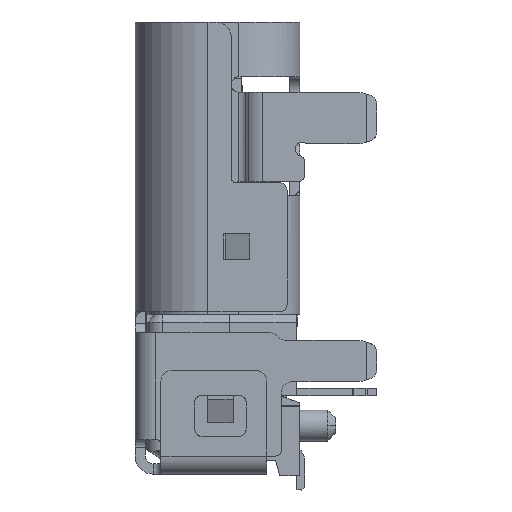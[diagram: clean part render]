
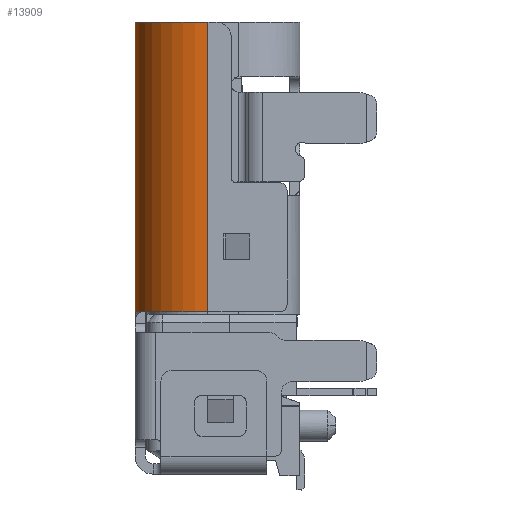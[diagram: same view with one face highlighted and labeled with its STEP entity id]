
A CAD part, left-side view. The second image highlights one B-rep face of the part: STEP entity #13909.
In plain terms, the highlighted cylindrical face has radius 1.41 mm (diameter 2.82 mm), a partial arc.
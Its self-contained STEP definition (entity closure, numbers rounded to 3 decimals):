
#356 = CYLINDRICAL_SURFACE ( 'NONE', #32464, 1.41 ) ;
#725 = CIRCLE ( 'NONE', #54226, 1.41 ) ;
#740 = VECTOR ( 'NONE', #38979, 1000. ) ;
#6155 = ORIENTED_EDGE ( 'NONE', *, *, #52917, .T. ) ;
#6172 = EDGE_CURVE ( 'NONE', #33294, #39685, #14687, .T. ) ;
#8142 = DIRECTION ( 'NONE',  ( 0., 0., 1. ) ) ;
#9703 = ORIENTED_EDGE ( 'NONE', *, *, #45828, .F. ) ;
#11877 = CARTESIAN_POINT ( 'NONE',  ( -360.4, -0.3, -255.061 ) ) ;
#13909 = ADVANCED_FACE ( 'NONE', ( #19484 ), #356, .T. ) ;
#14687 = LINE ( 'NONE', #74076, #740 ) ;
#17367 = LINE ( 'NONE', #78723, #37269 ) ;
#19484 = FACE_OUTER_BOUND ( 'NONE', #42859, .T. ) ;
#20336 = CARTESIAN_POINT ( 'NONE',  ( -361.81, -0.3, -249.451 ) ) ;
#21055 = EDGE_CURVE ( 'NONE', #33294, #36418, #49815, .T. ) ;
#22027 = VERTEX_POINT ( 'NONE', #27323 ) ;
#25680 = DIRECTION ( 'NONE',  ( 1., 0., 0. ) ) ;
#27323 = CARTESIAN_POINT ( 'NONE',  ( -360.4, -0.3, -249.451 ) ) ;
#29666 = DIRECTION ( 'NONE',  ( 0., 0., 1. ) ) ;
#31049 = DIRECTION ( 'NONE',  ( 1., 0., 0. ) ) ;
#32464 = AXIS2_PLACEMENT_3D ( 'NONE', #43777, #37000, #31049 ) ;
#33294 = VERTEX_POINT ( 'NONE', #44863 ) ;
#36418 = VERTEX_POINT ( 'NONE', #11877 ) ;
#37000 = DIRECTION ( 'NONE',  ( 0., 0., 1. ) ) ;
#37269 = VECTOR ( 'NONE', #29666, 1000. ) ;
#38299 = CARTESIAN_POINT ( 'NONE',  ( -361.81, -1.71, -249.451 ) ) ;
#38979 = DIRECTION ( 'NONE',  ( 0., 0., 1. ) ) ;
#39685 = VERTEX_POINT ( 'NONE', #38299 ) ;
#42859 = EDGE_LOOP ( 'NONE', ( #9703, #61180, #71038, #6155 ) ) ;
#43777 = CARTESIAN_POINT ( 'NONE',  ( -361.81, -0.3, -255.223 ) ) ;
#44611 = DIRECTION ( 'NONE',  ( 1., 0., 0. ) ) ;
#44863 = CARTESIAN_POINT ( 'NONE',  ( -361.81, -1.71, -255.061 ) ) ;
#45828 = EDGE_CURVE ( 'NONE', #39685, #22027, #725, .T. ) ;
#49815 = CIRCLE ( 'NONE', #63832, 1.41 ) ;
#52917 = EDGE_CURVE ( 'NONE', #36418, #22027, #17367, .T. ) ;
#54226 = AXIS2_PLACEMENT_3D ( 'NONE', #20336, #62595, #44611 ) ;
#61180 = ORIENTED_EDGE ( 'NONE', *, *, #6172, .F. ) ;
#62595 = DIRECTION ( 'NONE',  ( 0., 0., 1. ) ) ;
#62753 = CARTESIAN_POINT ( 'NONE',  ( -361.81, -0.3, -255.061 ) ) ;
#63832 = AXIS2_PLACEMENT_3D ( 'NONE', #62753, #8142, #25680 ) ;
#71038 = ORIENTED_EDGE ( 'NONE', *, *, #21055, .T. ) ;
#74076 = CARTESIAN_POINT ( 'NONE',  ( -361.81, -1.71, -249.218 ) ) ;
#78723 = CARTESIAN_POINT ( 'NONE',  ( -360.4, -0.3, -255.223 ) ) ;
